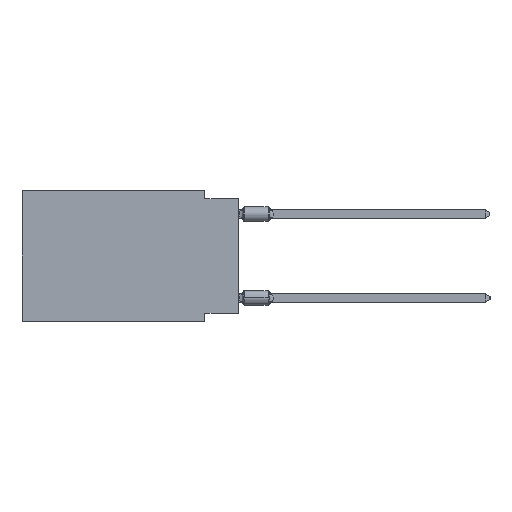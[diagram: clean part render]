
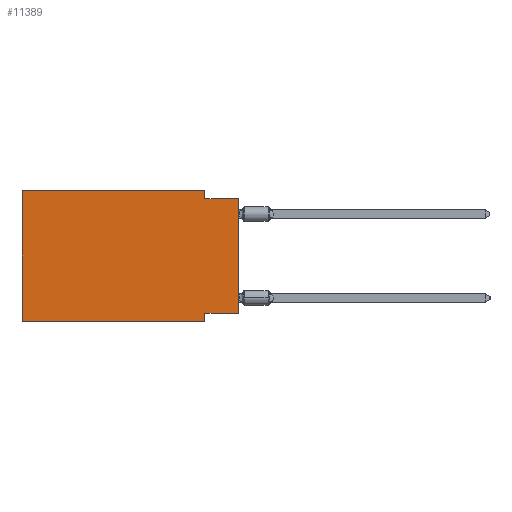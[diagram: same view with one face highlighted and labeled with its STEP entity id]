
A CAD part, left-side view. The second image highlights one B-rep face of the part: STEP entity #11389.
In plain terms, the highlighted planar face has unit normal (-1, 0, 0).
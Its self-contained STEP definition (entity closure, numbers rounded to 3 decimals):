
#191 = LINE ( 'NONE', #7251, #38891 ) ;
#881 = PLANE ( 'NONE',  #16784 ) ;
#1320 = DIRECTION ( 'NONE',  ( 0., -1., 0. ) ) ;
#1890 = DIRECTION ( 'NONE',  ( 0., 0., 1. ) ) ;
#1959 = DIRECTION ( 'NONE',  ( 0., 0., -1. ) ) ;
#2634 = LINE ( 'NONE', #25956, #40843 ) ;
#3361 = CARTESIAN_POINT ( 'NONE',  ( 0., 2.54, -9.271 ) ) ;
#3931 = VERTEX_POINT ( 'NONE', #26770 ) ;
#4867 = DIRECTION ( 'NONE',  ( 0., 0., 1. ) ) ;
#6119 = CARTESIAN_POINT ( 'NONE',  ( 0., 2.54, -0.635 ) ) ;
#6834 = CARTESIAN_POINT ( 'NONE',  ( 0., 16.383, 0. ) ) ;
#7251 = CARTESIAN_POINT ( 'NONE',  ( 0., 0., -0.635 ) ) ;
#7600 = CARTESIAN_POINT ( 'NONE',  ( 0., 2.54, 0. ) ) ;
#8089 = ORIENTED_EDGE ( 'NONE', *, *, #38836, .F. ) ;
#9250 = VECTOR ( 'NONE', #4867, 1000. ) ;
#9519 = VERTEX_POINT ( 'NONE', #21324 ) ;
#9915 = ORIENTED_EDGE ( 'NONE', *, *, #16959, .F. ) ;
#10491 = VERTEX_POINT ( 'NONE', #29701 ) ;
#11389 = ADVANCED_FACE ( 'NONE', ( #30235 ), #881, .F. ) ;
#11596 = CARTESIAN_POINT ( 'NONE',  ( 0., 16.383, 0. ) ) ;
#12651 = LINE ( 'NONE', #31740, #16188 ) ;
#12964 = VERTEX_POINT ( 'NONE', #6834 ) ;
#12972 = VECTOR ( 'NONE', #30605, 1000. ) ;
#13644 = VERTEX_POINT ( 'NONE', #6119 ) ;
#13809 = CARTESIAN_POINT ( 'NONE',  ( 0., 16.383, -9.906 ) ) ;
#14296 = CARTESIAN_POINT ( 'NONE',  ( 0., 16.383, 0. ) ) ;
#15137 = EDGE_CURVE ( 'NONE', #28431, #13644, #2634, .T. ) ;
#16188 = VECTOR ( 'NONE', #25719, 1000. ) ;
#16784 = AXIS2_PLACEMENT_3D ( 'NONE', #27031, #40131, #1959 ) ;
#16894 = DIRECTION ( 'NONE',  ( 0., -1., 0. ) ) ;
#16959 = EDGE_CURVE ( 'NONE', #13644, #3931, #191, .T. ) ;
#18238 = ORIENTED_EDGE ( 'NONE', *, *, #37256, .T. ) ;
#18401 = VECTOR ( 'NONE', #30023, 1000. ) ;
#19166 = EDGE_CURVE ( 'NONE', #10491, #34604, #20513, .T. ) ;
#19723 = CARTESIAN_POINT ( 'NONE',  ( 0., 16.383, -9.906 ) ) ;
#19826 = EDGE_CURVE ( 'NONE', #30942, #9519, #29590, .T. ) ;
#20513 = LINE ( 'NONE', #33819, #12972 ) ;
#21132 = LINE ( 'NONE', #34231, #9250 ) ;
#21324 = CARTESIAN_POINT ( 'NONE',  ( 0., 2.54, -9.906 ) ) ;
#22933 = DIRECTION ( 'NONE',  ( 0., 0., -1. ) ) ;
#23514 = ORIENTED_EDGE ( 'NONE', *, *, #15137, .F. ) ;
#23601 = VECTOR ( 'NONE', #1320, 1000. ) ;
#25719 = DIRECTION ( 'NONE',  ( 0., 0., -1. ) ) ;
#25956 = CARTESIAN_POINT ( 'NONE',  ( 0., 2.54, 0. ) ) ;
#26242 = EDGE_LOOP ( 'NONE', ( #18238, #9915, #23514, #27572, #41384, #37284, #8089, #30690 ) ) ;
#26770 = CARTESIAN_POINT ( 'NONE',  ( 0., 0., -0.635 ) ) ;
#27031 = CARTESIAN_POINT ( 'NONE',  ( 0., 16.383, 0. ) ) ;
#27572 = ORIENTED_EDGE ( 'NONE', *, *, #33897, .F. ) ;
#28055 = EDGE_CURVE ( 'NONE', #30942, #12964, #40926, .T. ) ;
#28431 = VERTEX_POINT ( 'NONE', #7600 ) ;
#29590 = LINE ( 'NONE', #19723, #18401 ) ;
#29701 = CARTESIAN_POINT ( 'NONE',  ( 0., 0., -9.271 ) ) ;
#30023 = DIRECTION ( 'NONE',  ( 0., -1., 0. ) ) ;
#30235 = FACE_OUTER_BOUND ( 'NONE', #26242, .T. ) ;
#30605 = DIRECTION ( 'NONE',  ( 0., 1., 0. ) ) ;
#30690 = ORIENTED_EDGE ( 'NONE', *, *, #19166, .F. ) ;
#30942 = VERTEX_POINT ( 'NONE', #13809 ) ;
#31520 = LINE ( 'NONE', #11596, #23601 ) ;
#31740 = CARTESIAN_POINT ( 'NONE',  ( 0., 2.54, -9.906 ) ) ;
#33819 = CARTESIAN_POINT ( 'NONE',  ( 0., 0., -9.271 ) ) ;
#33897 = EDGE_CURVE ( 'NONE', #12964, #28431, #31520, .T. ) ;
#34231 = CARTESIAN_POINT ( 'NONE',  ( 0., 0., 0. ) ) ;
#34604 = VERTEX_POINT ( 'NONE', #3361 ) ;
#37256 = EDGE_CURVE ( 'NONE', #10491, #3931, #21132, .T. ) ;
#37284 = ORIENTED_EDGE ( 'NONE', *, *, #19826, .T. ) ;
#38757 = VECTOR ( 'NONE', #1890, 1000. ) ;
#38836 = EDGE_CURVE ( 'NONE', #34604, #9519, #12651, .T. ) ;
#38891 = VECTOR ( 'NONE', #16894, 1000. ) ;
#40131 = DIRECTION ( 'NONE',  ( 1., 0., 0. ) ) ;
#40843 = VECTOR ( 'NONE', #22933, 1000. ) ;
#40926 = LINE ( 'NONE', #14296, #38757 ) ;
#41384 = ORIENTED_EDGE ( 'NONE', *, *, #28055, .F. ) ;
